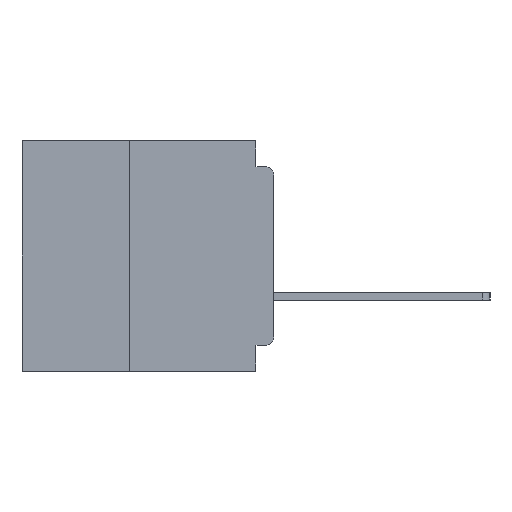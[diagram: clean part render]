
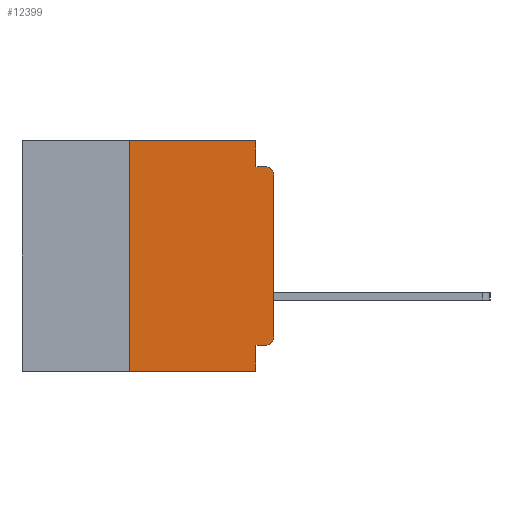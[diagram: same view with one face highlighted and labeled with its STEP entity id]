
A CAD part, left-side view. The second image highlights one B-rep face of the part: STEP entity #12399.
In plain terms, the highlighted planar face has unit normal (-1, 0, 0).
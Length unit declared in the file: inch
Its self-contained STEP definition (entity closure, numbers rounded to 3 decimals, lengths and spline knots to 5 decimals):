
#503 = AXIS2_PLACEMENT_3D ( 'NONE', #17736, #44452, #21616 ) ;
#1369 = CARTESIAN_POINT ( 'NONE',  ( 0., 0.437, -0.4 ) ) ;
#1643 = EDGE_CURVE ( 'NONE', #32576, #13967, #28515, .T. ) ;
#2289 = LINE ( 'NONE', #33384, #20378 ) ;
#2813 = ORIENTED_EDGE ( 'NONE', *, *, #11124, .T. ) ;
#3163 = CARTESIAN_POINT ( 'NONE',  ( 0., 0.015, -0.355 ) ) ;
#4178 = FACE_OUTER_BOUND ( 'NONE', #23022, .T. ) ;
#4573 = EDGE_CURVE ( 'NONE', #24688, #22793, #9633, .T. ) ;
#5191 = DIRECTION ( 'NONE',  ( 0., -1., 0. ) ) ;
#5222 = EDGE_CURVE ( 'NONE', #29287, #9190, #8962, .T. ) ;
#5231 = DIRECTION ( 'NONE',  ( -1., 0., 0. ) ) ;
#6034 = EDGE_CURVE ( 'NONE', #12469, #23665, #2289, .T. ) ;
#6076 = LINE ( 'NONE', #12076, #24202 ) ;
#6139 = ORIENTED_EDGE ( 'NONE', *, *, #39390, .T. ) ;
#6205 = DIRECTION ( 'NONE',  ( 0., 0., 1. ) ) ;
#7479 = CARTESIAN_POINT ( 'NONE',  ( 0., 0.437, 0. ) ) ;
#7706 = EDGE_CURVE ( 'NONE', #16281, #45618, #14219, .T. ) ;
#8150 = LINE ( 'NONE', #17710, #27503 ) ;
#8962 = LINE ( 'NONE', #28610, #38427 ) ;
#9190 = VERTEX_POINT ( 'NONE', #30789 ) ;
#9343 = CARTESIAN_POINT ( 'NONE',  ( 0., 0.031, 0. ) ) ;
#9357 = ORIENTED_EDGE ( 'NONE', *, *, #5222, .F. ) ;
#9506 = ORIENTED_EDGE ( 'NONE', *, *, #15280, .F. ) ;
#9633 = CIRCLE ( 'NONE', #34350, 0.015 ) ;
#11124 = EDGE_CURVE ( 'NONE', #29287, #23665, #43225, .T. ) ;
#11860 = CARTESIAN_POINT ( 'NONE',  ( 0., 0.015, -0.045 ) ) ;
#12076 = CARTESIAN_POINT ( 'NONE',  ( 0., 0., -0.045 ) ) ;
#12399 = ADVANCED_FACE ( 'NONE', ( #4178 ), #33034, .F. ) ;
#12469 = VERTEX_POINT ( 'NONE', #37318 ) ;
#12656 = VECTOR ( 'NONE', #45704, 39.37008 ) ;
#12802 = CARTESIAN_POINT ( 'NONE',  ( 0., 0.25, -0.4 ) ) ;
#13233 = DIRECTION ( 'NONE',  ( 0., 0., -1. ) ) ;
#13967 = VERTEX_POINT ( 'NONE', #11860 ) ;
#14219 = LINE ( 'NONE', #9343, #42371 ) ;
#15204 = CARTESIAN_POINT ( 'NONE',  ( 0., 0.031, -0.045 ) ) ;
#15280 = EDGE_CURVE ( 'NONE', #45618, #13967, #6076, .T. ) ;
#15760 = EDGE_CURVE ( 'NONE', #9190, #16281, #26575, .T. ) ;
#16281 = VERTEX_POINT ( 'NONE', #42079 ) ;
#16893 = DIRECTION ( 'NONE',  ( -1., 0., 0. ) ) ;
#16958 = DIRECTION ( 'NONE',  ( 0., 1., 0. ) ) ;
#17710 = CARTESIAN_POINT ( 'NONE',  ( 0., 0., 0. ) ) ;
#17736 = CARTESIAN_POINT ( 'NONE',  ( 0., 0.437, 0. ) ) ;
#18401 = CARTESIAN_POINT ( 'NONE',  ( 0., 0., -0.06 ) ) ;
#20270 = CARTESIAN_POINT ( 'NONE',  ( 0., 0., -0.34 ) ) ;
#20378 = VECTOR ( 'NONE', #37173, 39.37008 ) ;
#21616 = DIRECTION ( 'NONE',  ( 0., 0., -1. ) ) ;
#22793 = VERTEX_POINT ( 'NONE', #20270 ) ;
#23022 = EDGE_LOOP ( 'NONE', ( #6139, #43632, #9506, #27036, #31074, #9357, #2813, #47512, #28349, #28615 ) ) ;
#23665 = VERTEX_POINT ( 'NONE', #44863 ) ;
#24202 = VECTOR ( 'NONE', #38952, 39.37008 ) ;
#24688 = VERTEX_POINT ( 'NONE', #3163 ) ;
#25020 = EDGE_CURVE ( 'NONE', #24688, #12469, #38902, .T. ) ;
#26575 = LINE ( 'NONE', #7479, #12656 ) ;
#27036 = ORIENTED_EDGE ( 'NONE', *, *, #7706, .F. ) ;
#27503 = VECTOR ( 'NONE', #6205, 39.37008 ) ;
#28340 = CARTESIAN_POINT ( 'NONE',  ( 0., 0.015, -0.34 ) ) ;
#28349 = ORIENTED_EDGE ( 'NONE', *, *, #25020, .F. ) ;
#28515 = CIRCLE ( 'NONE', #38720, 0.015 ) ;
#28610 = CARTESIAN_POINT ( 'NONE',  ( 0., 0.25, -0.4 ) ) ;
#28615 = ORIENTED_EDGE ( 'NONE', *, *, #4573, .T. ) ;
#29287 = VERTEX_POINT ( 'NONE', #12802 ) ;
#30789 = CARTESIAN_POINT ( 'NONE',  ( 0., 0.25, 0. ) ) ;
#31074 = ORIENTED_EDGE ( 'NONE', *, *, #15760, .F. ) ;
#32187 = DIRECTION ( 'NONE',  ( 0., 0., -1. ) ) ;
#32576 = VERTEX_POINT ( 'NONE', #18401 ) ;
#33034 = PLANE ( 'NONE',  #503 ) ;
#33157 = VECTOR ( 'NONE', #5191, 39.37008 ) ;
#33384 = CARTESIAN_POINT ( 'NONE',  ( 0., 0.031, -0.4 ) ) ;
#34350 = AXIS2_PLACEMENT_3D ( 'NONE', #28340, #5231, #32187 ) ;
#37173 = DIRECTION ( 'NONE',  ( 0., 0., -1. ) ) ;
#37318 = CARTESIAN_POINT ( 'NONE',  ( 0., 0.031, -0.355 ) ) ;
#38427 = VECTOR ( 'NONE', #47541, 39.37008 ) ;
#38720 = AXIS2_PLACEMENT_3D ( 'NONE', #39833, #16893, #43621 ) ;
#38902 = LINE ( 'NONE', #39910, #40103 ) ;
#38952 = DIRECTION ( 'NONE',  ( 0., -1., 0. ) ) ;
#39390 = EDGE_CURVE ( 'NONE', #22793, #32576, #8150, .T. ) ;
#39833 = CARTESIAN_POINT ( 'NONE',  ( 0., 0.015, -0.06 ) ) ;
#39910 = CARTESIAN_POINT ( 'NONE',  ( 0., 0., -0.355 ) ) ;
#40103 = VECTOR ( 'NONE', #16958, 39.37008 ) ;
#42079 = CARTESIAN_POINT ( 'NONE',  ( 0., 0.031, 0. ) ) ;
#42371 = VECTOR ( 'NONE', #13233, 39.37008 ) ;
#43225 = LINE ( 'NONE', #1369, #33157 ) ;
#43621 = DIRECTION ( 'NONE',  ( 0., 0., -1. ) ) ;
#43632 = ORIENTED_EDGE ( 'NONE', *, *, #1643, .T. ) ;
#44452 = DIRECTION ( 'NONE',  ( 1., 0., 0. ) ) ;
#44863 = CARTESIAN_POINT ( 'NONE',  ( 0., 0.031, -0.4 ) ) ;
#45618 = VERTEX_POINT ( 'NONE', #15204 ) ;
#45704 = DIRECTION ( 'NONE',  ( 0., -1., 0. ) ) ;
#47512 = ORIENTED_EDGE ( 'NONE', *, *, #6034, .F. ) ;
#47541 = DIRECTION ( 'NONE',  ( 0., 0., 1. ) ) ;
